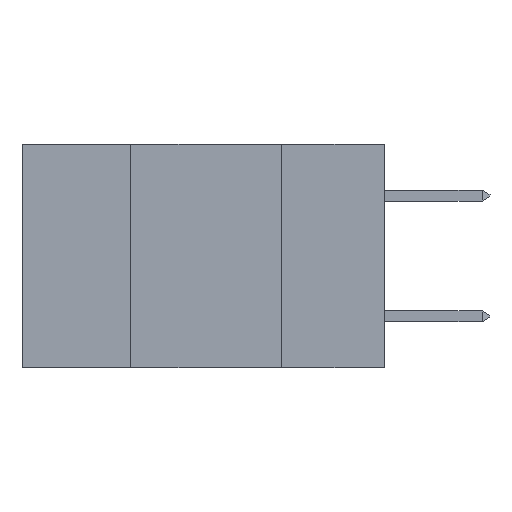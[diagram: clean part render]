
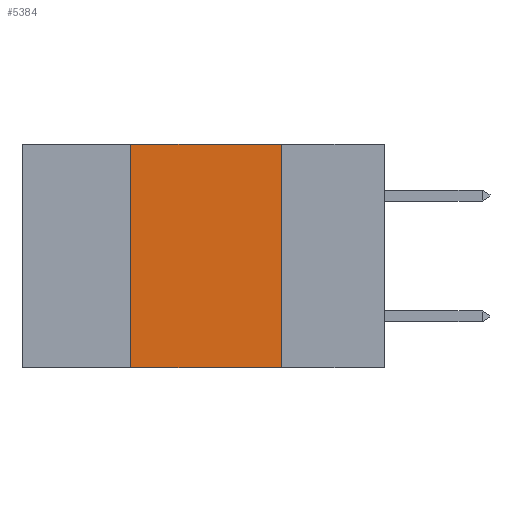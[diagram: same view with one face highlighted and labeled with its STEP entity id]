
A CAD part, left-side view. The second image highlights one B-rep face of the part: STEP entity #5384.
In plain terms, the highlighted planar face has unit normal (-1, 0, 0).
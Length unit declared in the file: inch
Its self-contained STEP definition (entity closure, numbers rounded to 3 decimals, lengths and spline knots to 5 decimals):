
#253 = VERTEX_POINT ( 'NONE', #2969 ) ;
#383 = EDGE_CURVE ( 'NONE', #253, #8893, #4368, .T. ) ;
#572 = CARTESIAN_POINT ( 'NONE',  ( 0., 0.17, -0.37 ) ) ;
#598 = EDGE_CURVE ( 'NONE', #6278, #7793, #7898, .T. ) ;
#1134 = VECTOR ( 'NONE', #6720, 39.37008 ) ;
#1717 = PLANE ( 'NONE',  #10475 ) ;
#2025 = ORIENTED_EDGE ( 'NONE', *, *, #9103, .F. ) ;
#2032 = VECTOR ( 'NONE', #3638, 39.37008 ) ;
#2546 = DIRECTION ( 'NONE',  ( 1., 0., 0. ) ) ;
#2783 = CARTESIAN_POINT ( 'NONE',  ( 0., 0.42, 0. ) ) ;
#2969 = CARTESIAN_POINT ( 'NONE',  ( 0., 0.42, 0. ) ) ;
#3638 = DIRECTION ( 'NONE',  ( 0., 0., 1. ) ) ;
#4043 = VECTOR ( 'NONE', #10294, 39.37008 ) ;
#4297 = CARTESIAN_POINT ( 'NONE',  ( 0., 0.17, 0. ) ) ;
#4359 = LINE ( 'NONE', #2783, #2032 ) ;
#4368 = LINE ( 'NONE', #6378, #4043 ) ;
#4958 = VECTOR ( 'NONE', #6039, 39.37008 ) ;
#5384 = ADVANCED_FACE ( 'NONE', ( #10022 ), #1717, .F. ) ;
#5601 = CARTESIAN_POINT ( 'NONE',  ( 0., 0.6, -0.37 ) ) ;
#6027 = CARTESIAN_POINT ( 'NONE',  ( 0., 0.6, 0. ) ) ;
#6039 = DIRECTION ( 'NONE',  ( 0., 0., -1. ) ) ;
#6278 = VERTEX_POINT ( 'NONE', #9198 ) ;
#6378 = CARTESIAN_POINT ( 'NONE',  ( 0., 0.6, 0. ) ) ;
#6720 = DIRECTION ( 'NONE',  ( 0., -1., 0. ) ) ;
#7135 = LINE ( 'NONE', #4297, #4958 ) ;
#7793 = VERTEX_POINT ( 'NONE', #572 ) ;
#7898 = LINE ( 'NONE', #5601, #1134 ) ;
#8443 = DIRECTION ( 'NONE',  ( 0., 0., -1. ) ) ;
#8703 = ORIENTED_EDGE ( 'NONE', *, *, #598, .T. ) ;
#8893 = VERTEX_POINT ( 'NONE', #10282 ) ;
#9103 = EDGE_CURVE ( 'NONE', #8893, #7793, #7135, .T. ) ;
#9198 = CARTESIAN_POINT ( 'NONE',  ( 0., 0.42, -0.37 ) ) ;
#9529 = EDGE_LOOP ( 'NONE', ( #2025, #10348, #10319, #8703 ) ) ;
#10022 = FACE_OUTER_BOUND ( 'NONE', #9529, .T. ) ;
#10282 = CARTESIAN_POINT ( 'NONE',  ( 0., 0.17, 0. ) ) ;
#10294 = DIRECTION ( 'NONE',  ( 0., -1., 0. ) ) ;
#10319 = ORIENTED_EDGE ( 'NONE', *, *, #10470, .F. ) ;
#10348 = ORIENTED_EDGE ( 'NONE', *, *, #383, .F. ) ;
#10470 = EDGE_CURVE ( 'NONE', #6278, #253, #4359, .T. ) ;
#10475 = AXIS2_PLACEMENT_3D ( 'NONE', #6027, #2546, #8443 ) ;
